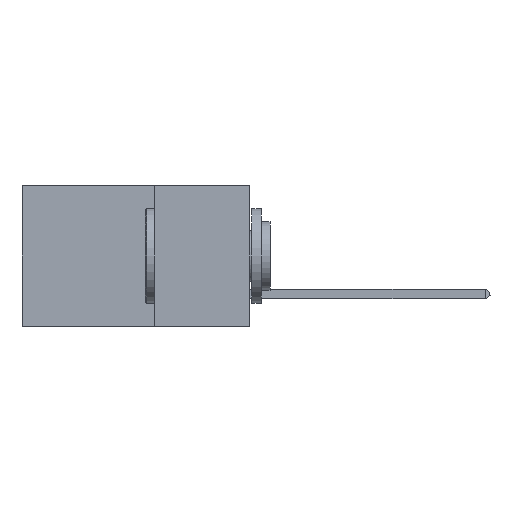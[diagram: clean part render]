
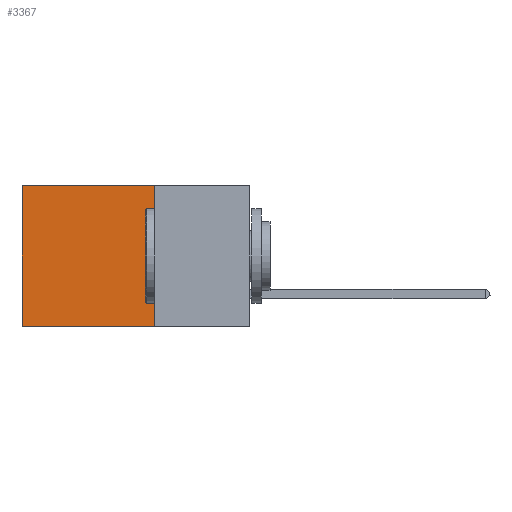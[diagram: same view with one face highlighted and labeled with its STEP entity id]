
A CAD part, left-side view. The second image highlights one B-rep face of the part: STEP entity #3367.
In plain terms, the highlighted planar face has unit normal (-1, 0, 0).
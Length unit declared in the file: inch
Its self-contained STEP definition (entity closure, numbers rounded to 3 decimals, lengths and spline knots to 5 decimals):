
#418 = DIRECTION ( 'NONE',  ( 1., 0., 0. ) ) ;
#724 = LINE ( 'NONE', #37859, #33418 ) ;
#2451 = EDGE_CURVE ( 'NONE', #25227, #26633, #35261, .T. ) ;
#3367 = ADVANCED_FACE ( 'NONE', ( #7945 ), #28372, .F. ) ;
#3545 = ORIENTED_EDGE ( 'NONE', *, *, #28996, .F. ) ;
#3832 = ORIENTED_EDGE ( 'NONE', *, *, #9253, .T. ) ;
#4122 = VECTOR ( 'NONE', #6372, 39.37008 ) ;
#6372 = DIRECTION ( 'NONE',  ( 0., 0., -1. ) ) ;
#7945 = FACE_OUTER_BOUND ( 'NONE', #36112, .T. ) ;
#8257 = LINE ( 'NONE', #27505, #37946 ) ;
#8707 = VERTEX_POINT ( 'NONE', #22620 ) ;
#9155 = CARTESIAN_POINT ( 'NONE',  ( 0.2875, 0.6, 0. ) ) ;
#9207 = CARTESIAN_POINT ( 'NONE',  ( 0.2875, 0.6, 0. ) ) ;
#9253 = EDGE_CURVE ( 'NONE', #26633, #8707, #38219, .T. ) ;
#11868 = VECTOR ( 'NONE', #27575, 39.37008 ) ;
#19025 = CARTESIAN_POINT ( 'NONE',  ( 0.2875, 0.25, 0. ) ) ;
#22208 = DIRECTION ( 'NONE',  ( 0., 0., -1. ) ) ;
#22620 = CARTESIAN_POINT ( 'NONE',  ( 0.2875, 0.6, -0.37 ) ) ;
#22747 = ORIENTED_EDGE ( 'NONE', *, *, #2451, .T. ) ;
#24861 = CARTESIAN_POINT ( 'NONE',  ( 0.2875, 0.25, 0. ) ) ;
#25227 = VERTEX_POINT ( 'NONE', #24861 ) ;
#26633 = VERTEX_POINT ( 'NONE', #9207 ) ;
#27505 = CARTESIAN_POINT ( 'NONE',  ( 0.2875, 0.25, 0. ) ) ;
#27575 = DIRECTION ( 'NONE',  ( 0., 1., 0. ) ) ;
#28372 = PLANE ( 'NONE',  #36920 ) ;
#28996 = EDGE_CURVE ( 'NONE', #25227, #35402, #8257, .T. ) ;
#30544 = CARTESIAN_POINT ( 'NONE',  ( 0.2875, 0.25, 0. ) ) ;
#31714 = EDGE_CURVE ( 'NONE', #35402, #8707, #724, .T. ) ;
#33226 = CARTESIAN_POINT ( 'NONE',  ( 0.2875, 0.25, -0.37 ) ) ;
#33418 = VECTOR ( 'NONE', #37467, 39.37008 ) ;
#35097 = ORIENTED_EDGE ( 'NONE', *, *, #31714, .F. ) ;
#35261 = LINE ( 'NONE', #30544, #11868 ) ;
#35402 = VERTEX_POINT ( 'NONE', #33226 ) ;
#36112 = EDGE_LOOP ( 'NONE', ( #3832, #35097, #3545, #22747 ) ) ;
#36920 = AXIS2_PLACEMENT_3D ( 'NONE', #19025, #418, #22208 ) ;
#37467 = DIRECTION ( 'NONE',  ( 0., 1., 0. ) ) ;
#37859 = CARTESIAN_POINT ( 'NONE',  ( 0.2875, 0.25, -0.37 ) ) ;
#37946 = VECTOR ( 'NONE', #40218, 39.37008 ) ;
#38219 = LINE ( 'NONE', #9155, #4122 ) ;
#40218 = DIRECTION ( 'NONE',  ( 0., 0., -1. ) ) ;
